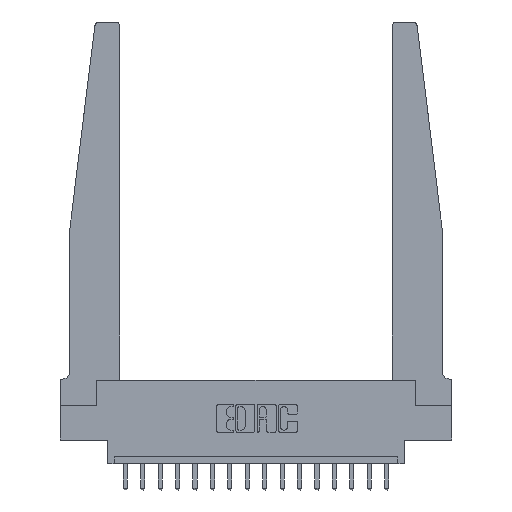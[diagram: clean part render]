
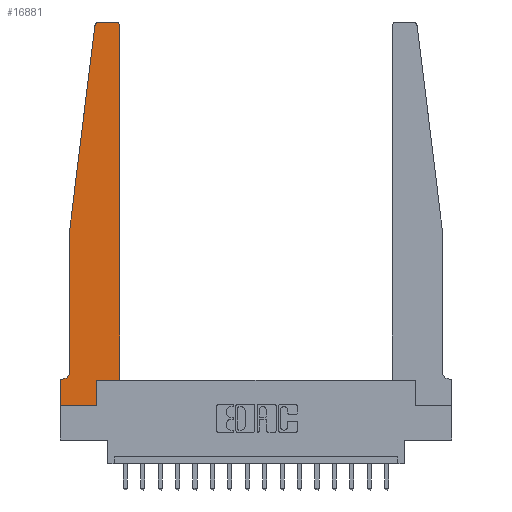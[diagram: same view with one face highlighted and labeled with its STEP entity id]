
A CAD part, top view. The second image highlights one B-rep face of the part: STEP entity #16881.
In plain terms, the highlighted planar face has unit normal (0, 0, 1).
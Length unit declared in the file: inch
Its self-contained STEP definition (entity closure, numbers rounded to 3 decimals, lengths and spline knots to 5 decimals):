
#320 = EDGE_CURVE ( 'NONE', #7214, #8052, #12861, .T. ) ;
#414 = VECTOR ( 'NONE', #12273, 39.37008 ) ;
#620 = DIRECTION ( 'NONE',  ( 1., 0., 0. ) ) ;
#692 = LINE ( 'NONE', #15429, #17809 ) ;
#711 = VERTEX_POINT ( 'NONE', #8632 ) ;
#1192 = CIRCLE ( 'NONE', #13324, 0.03 ) ;
#1351 = EDGE_CURVE ( 'NONE', #7132, #7214, #1192, .T. ) ;
#1406 = EDGE_CURVE ( 'NONE', #3586, #6303, #8270, .T. ) ;
#2111 = CARTESIAN_POINT ( 'NONE',  ( 0.27653, 2.72, 0.37 ) ) ;
#2281 = DIRECTION ( 'NONE',  ( 0., 0., 1. ) ) ;
#2442 = EDGE_CURVE ( 'NONE', #711, #4183, #14524, .T. ) ;
#2600 = ORIENTED_EDGE ( 'NONE', *, *, #1406, .T. ) ;
#2713 = CARTESIAN_POINT ( 'NONE',  ( 0., 0.1875, 0.37 ) ) ;
#2848 = VERTEX_POINT ( 'NONE', #4208 ) ;
#3183 = CARTESIAN_POINT ( 'NONE',  ( 0., 0., 0.37 ) ) ;
#3184 = VERTEX_POINT ( 'NONE', #6933 ) ;
#3288 = DIRECTION ( 'NONE',  ( -1., 0., 0. ) ) ;
#3531 = EDGE_CURVE ( 'NONE', #5398, #3184, #8798, .T. ) ;
#3586 = VERTEX_POINT ( 'NONE', #15767 ) ;
#3697 = CARTESIAN_POINT ( 'NONE',  ( 0., 0., 0.37 ) ) ;
#3824 = DIRECTION ( 'NONE',  ( -1., 0., 0. ) ) ;
#4102 = VECTOR ( 'NONE', #18880, 39.37008 ) ;
#4183 = VERTEX_POINT ( 'NONE', #7626 ) ;
#4193 = ORIENTED_EDGE ( 'NONE', *, *, #16898, .T. ) ;
#4208 = CARTESIAN_POINT ( 'NONE',  ( 0.425, 0.18, 0.37 ) ) ;
#4236 = PLANE ( 'NONE',  #17483 ) ;
#4435 = ORIENTED_EDGE ( 'NONE', *, *, #16217, .T. ) ;
#4657 = CIRCLE ( 'NONE', #7980, 0.03 ) ;
#4730 = CARTESIAN_POINT ( 'NONE',  ( 0.425, 0.18, 0.37 ) ) ;
#4802 = VECTOR ( 'NONE', #12823, 39.37008 ) ;
#4992 = VECTOR ( 'NONE', #3824, 39.37008 ) ;
#5012 = ORIENTED_EDGE ( 'NONE', *, *, #13737, .T. ) ;
#5131 = DIRECTION ( 'NONE',  ( -1., 0., 0. ) ) ;
#5319 = VECTOR ( 'NONE', #16367, 39.37008 ) ;
#5398 = VERTEX_POINT ( 'NONE', #12019 ) ;
#5523 = CARTESIAN_POINT ( 'NONE',  ( 0.2605, 0.18, 0.37 ) ) ;
#5536 = ORIENTED_EDGE ( 'NONE', *, *, #17368, .T. ) ;
#5879 = VECTOR ( 'NONE', #6410, 39.37008 ) ;
#6303 = VERTEX_POINT ( 'NONE', #10567 ) ;
#6410 = DIRECTION ( 'NONE',  ( 0., -1., 0. ) ) ;
#6547 = DIRECTION ( 'NONE',  ( 0., 0., -1. ) ) ;
#6575 = DIRECTION ( 'NONE',  ( 0., -1., 0. ) ) ;
#6646 = LINE ( 'NONE', #18244, #414 ) ;
#6673 = VECTOR ( 'NONE', #3288, 39.37008 ) ;
#6933 = CARTESIAN_POINT ( 'NONE',  ( 0.065, 1.25, 0.37 ) ) ;
#6943 = CARTESIAN_POINT ( 'NONE',  ( 0.395, 2.72, 0.37 ) ) ;
#6982 = CARTESIAN_POINT ( 'NONE',  ( 0.395, 2.75, 0.37 ) ) ;
#7071 = CIRCLE ( 'NONE', #13172, 0.05 ) ;
#7132 = VERTEX_POINT ( 'NONE', #16952 ) ;
#7214 = VERTEX_POINT ( 'NONE', #6982 ) ;
#7447 = DIRECTION ( 'NONE',  ( 0., 0., 1. ) ) ;
#7626 = CARTESIAN_POINT ( 'NONE',  ( 0., 0.1875, 0.37 ) ) ;
#7980 = AXIS2_PLACEMENT_3D ( 'NONE', #2111, #2281, #18044 ) ;
#8052 = VERTEX_POINT ( 'NONE', #17378 ) ;
#8270 = LINE ( 'NONE', #5523, #18562 ) ;
#8319 = EDGE_CURVE ( 'NONE', #15049, #3586, #15763, .T. ) ;
#8369 = DIRECTION ( 'NONE',  ( 0., 1., 0. ) ) ;
#8632 = CARTESIAN_POINT ( 'NONE',  ( 0.015, 0.1875, 0.37 ) ) ;
#8641 = ORIENTED_EDGE ( 'NONE', *, *, #3531, .T. ) ;
#8798 = LINE ( 'NONE', #13018, #4102 ) ;
#8923 = ORIENTED_EDGE ( 'NONE', *, *, #2442, .T. ) ;
#9903 = CARTESIAN_POINT ( 'NONE',  ( 0., 0., 0.37 ) ) ;
#9950 = DIRECTION ( 'NONE',  ( 0., 0., 1. ) ) ;
#10567 = CARTESIAN_POINT ( 'NONE',  ( 0.2605, 0.18, 0.37 ) ) ;
#10980 = VERTEX_POINT ( 'NONE', #15311 ) ;
#11370 = FACE_OUTER_BOUND ( 'NONE', #11559, .T. ) ;
#11559 = EDGE_LOOP ( 'NONE', ( #14130, #12015, #8641, #5536, #4435, #8923, #4193, #11704, #2600, #5012, #15017, #11732 ) ) ;
#11704 = ORIENTED_EDGE ( 'NONE', *, *, #8319, .T. ) ;
#11732 = ORIENTED_EDGE ( 'NONE', *, *, #1351, .T. ) ;
#11832 = CARTESIAN_POINT ( 'NONE',  ( 0.065, 0.1875, 0.37 ) ) ;
#12015 = ORIENTED_EDGE ( 'NONE', *, *, #13790, .T. ) ;
#12019 = CARTESIAN_POINT ( 'NONE',  ( 0.24675, 2.72367, 0.37 ) ) ;
#12273 = DIRECTION ( 'NONE',  ( 1., 0., 0. ) ) ;
#12772 = DIRECTION ( 'NONE',  ( 1., 0., 0. ) ) ;
#12823 = DIRECTION ( 'NONE',  ( 1., 0., 0. ) ) ;
#12861 = LINE ( 'NONE', #18726, #4992 ) ;
#13018 = CARTESIAN_POINT ( 'NONE',  ( 0.065, 1.25, 0.37 ) ) ;
#13172 = AXIS2_PLACEMENT_3D ( 'NONE', #14260, #6547, #5131 ) ;
#13324 = AXIS2_PLACEMENT_3D ( 'NONE', #6943, #9950, #12772 ) ;
#13737 = EDGE_CURVE ( 'NONE', #6303, #2848, #6646, .T. ) ;
#13790 = EDGE_CURVE ( 'NONE', #8052, #5398, #4657, .T. ) ;
#14130 = ORIENTED_EDGE ( 'NONE', *, *, #320, .T. ) ;
#14260 = CARTESIAN_POINT ( 'NONE',  ( 0.015, 0.2375, 0.37 ) ) ;
#14524 = LINE ( 'NONE', #11832, #6673 ) ;
#15017 = ORIENTED_EDGE ( 'NONE', *, *, #17790, .T. ) ;
#15049 = VERTEX_POINT ( 'NONE', #3697 ) ;
#15311 = CARTESIAN_POINT ( 'NONE',  ( 0.065, 0.2375, 0.37 ) ) ;
#15429 = CARTESIAN_POINT ( 'NONE',  ( 0.065, 1.25, 0.37 ) ) ;
#15763 = LINE ( 'NONE', #9903, #4802 ) ;
#15767 = CARTESIAN_POINT ( 'NONE',  ( 0.2605, 0., 0.37 ) ) ;
#16147 = LINE ( 'NONE', #3183, #5879 ) ;
#16217 = EDGE_CURVE ( 'NONE', #10980, #711, #7071, .T. ) ;
#16367 = DIRECTION ( 'NONE',  ( 0., 1., 0. ) ) ;
#16881 = ADVANCED_FACE ( 'NONE', ( #11370 ), #4236, .T. ) ;
#16898 = EDGE_CURVE ( 'NONE', #4183, #15049, #16147, .T. ) ;
#16952 = CARTESIAN_POINT ( 'NONE',  ( 0.425, 2.72, 0.37 ) ) ;
#17368 = EDGE_CURVE ( 'NONE', #3184, #10980, #692, .T. ) ;
#17378 = CARTESIAN_POINT ( 'NONE',  ( 0.27653, 2.75, 0.37 ) ) ;
#17483 = AXIS2_PLACEMENT_3D ( 'NONE', #2713, #7447, #620 ) ;
#17790 = EDGE_CURVE ( 'NONE', #2848, #7132, #17818, .T. ) ;
#17809 = VECTOR ( 'NONE', #6575, 39.37008 ) ;
#17818 = LINE ( 'NONE', #4730, #5319 ) ;
#18044 = DIRECTION ( 'NONE',  ( 1., 0., 0. ) ) ;
#18244 = CARTESIAN_POINT ( 'NONE',  ( 0.425, 0.18, 0.37 ) ) ;
#18562 = VECTOR ( 'NONE', #8369, 39.37008 ) ;
#18726 = CARTESIAN_POINT ( 'NONE',  ( 0.25, 2.75, 0.37 ) ) ;
#18880 = DIRECTION ( 'NONE',  ( -0.122, -0.992, 0. ) ) ;
